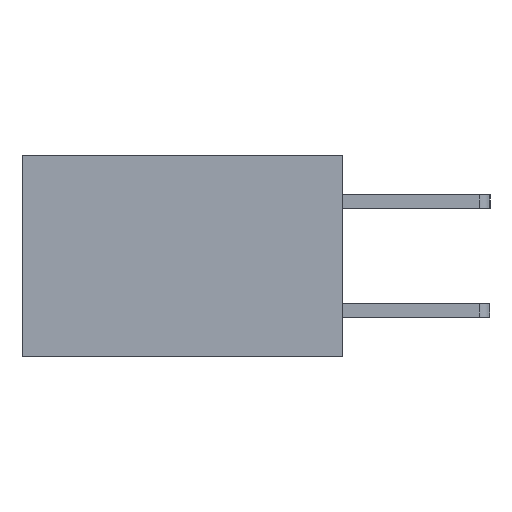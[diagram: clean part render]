
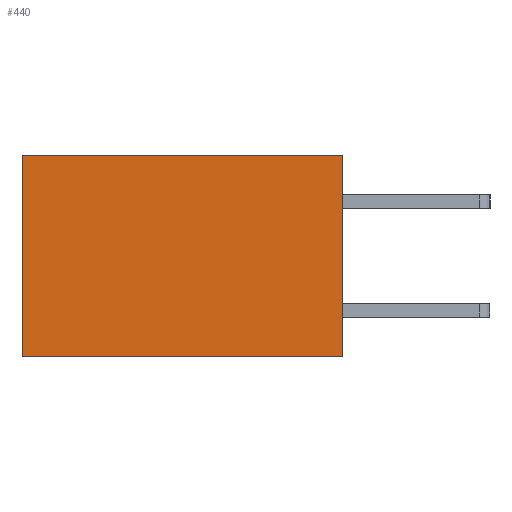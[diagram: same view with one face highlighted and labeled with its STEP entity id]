
A CAD part, left-side view. The second image highlights one B-rep face of the part: STEP entity #440.
In plain terms, the highlighted planar face has unit normal (-1, 0, 0).
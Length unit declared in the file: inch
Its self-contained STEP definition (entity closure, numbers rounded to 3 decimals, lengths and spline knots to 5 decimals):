
#112 = CARTESIAN_POINT ( 'NONE',  ( 0.277, 0., 0. ) ) ;
#440 = ADVANCED_FACE ( 'NONE', ( #1755 ), #13957, .F. ) ;
#592 = CARTESIAN_POINT ( 'NONE',  ( 0.277, 0., 0. ) ) ;
#1003 = DIRECTION ( 'NONE',  ( 0., 0., -1. ) ) ;
#1050 = VECTOR ( 'NONE', #6604, 39.37008 ) ;
#1641 = LINE ( 'NONE', #592, #10381 ) ;
#1755 = FACE_OUTER_BOUND ( 'NONE', #6113, .T. ) ;
#1868 = VECTOR ( 'NONE', #8465, 39.37008 ) ;
#1887 = CARTESIAN_POINT ( 'NONE',  ( 0.277, 0.59, -0.37 ) ) ;
#2282 = VERTEX_POINT ( 'NONE', #11157 ) ;
#2770 = VECTOR ( 'NONE', #1003, 39.37008 ) ;
#4010 = VERTEX_POINT ( 'NONE', #112 ) ;
#4873 = ORIENTED_EDGE ( 'NONE', *, *, #6203, .T. ) ;
#5050 = CARTESIAN_POINT ( 'NONE',  ( 0.277, 0.59, -0.37 ) ) ;
#5912 = LINE ( 'NONE', #11249, #2770 ) ;
#6113 = EDGE_LOOP ( 'NONE', ( #9276, #7179, #13070, #4873 ) ) ;
#6203 = EDGE_CURVE ( 'NONE', #4010, #14344, #1641, .T. ) ;
#6604 = DIRECTION ( 'NONE',  ( 0., 0., -1. ) ) ;
#6921 = LINE ( 'NONE', #1887, #1050 ) ;
#6954 = EDGE_CURVE ( 'NONE', #14344, #14603, #6921, .T. ) ;
#7179 = ORIENTED_EDGE ( 'NONE', *, *, #13284, .F. ) ;
#7344 = AXIS2_PLACEMENT_3D ( 'NONE', #7424, #12821, #12683 ) ;
#7424 = CARTESIAN_POINT ( 'NONE',  ( 0.277, 0., -0.37 ) ) ;
#7611 = DIRECTION ( 'NONE',  ( 0., 1., 0. ) ) ;
#8465 = DIRECTION ( 'NONE',  ( 0., 1., 0. ) ) ;
#9276 = ORIENTED_EDGE ( 'NONE', *, *, #6954, .T. ) ;
#9506 = CARTESIAN_POINT ( 'NONE',  ( 0.277, 0., -0.37 ) ) ;
#10173 = CARTESIAN_POINT ( 'NONE',  ( 0.277, 0.59, 0. ) ) ;
#10381 = VECTOR ( 'NONE', #7611, 39.37008 ) ;
#10940 = LINE ( 'NONE', #9506, #1868 ) ;
#11157 = CARTESIAN_POINT ( 'NONE',  ( 0.277, 0., -0.37 ) ) ;
#11249 = CARTESIAN_POINT ( 'NONE',  ( 0.277, 0., -0.37 ) ) ;
#12683 = DIRECTION ( 'NONE',  ( 0., 0., -1. ) ) ;
#12821 = DIRECTION ( 'NONE',  ( 1., 0., 0. ) ) ;
#13070 = ORIENTED_EDGE ( 'NONE', *, *, #14339, .F. ) ;
#13284 = EDGE_CURVE ( 'NONE', #2282, #14603, #10940, .T. ) ;
#13957 = PLANE ( 'NONE',  #7344 ) ;
#14339 = EDGE_CURVE ( 'NONE', #4010, #2282, #5912, .T. ) ;
#14344 = VERTEX_POINT ( 'NONE', #10173 ) ;
#14603 = VERTEX_POINT ( 'NONE', #5050 ) ;
